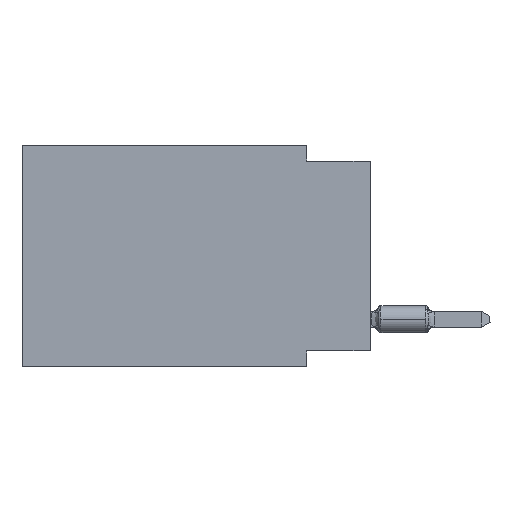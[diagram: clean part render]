
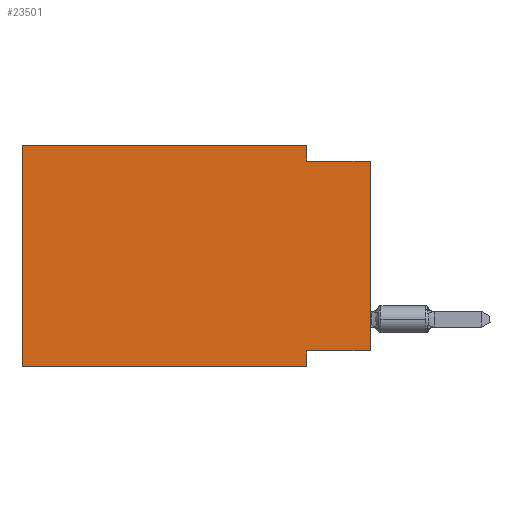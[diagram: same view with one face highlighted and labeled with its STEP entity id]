
A CAD part, left-side view. The second image highlights one B-rep face of the part: STEP entity #23501.
In plain terms, the highlighted planar face has unit normal (-1, 0, 0).
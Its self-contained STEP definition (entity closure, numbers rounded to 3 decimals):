
#1011 = DIRECTION ( 'NONE',  ( 0., -1., 0. ) ) ;
#1168 = DIRECTION ( 'NONE',  ( 0., -1., 0. ) ) ;
#1797 = FACE_OUTER_BOUND ( 'NONE', #10952, .T. ) ;
#2019 = ORIENTED_EDGE ( 'NONE', *, *, #16806, .T. ) ;
#2637 = CARTESIAN_POINT ( 'NONE',  ( 0., 2.54, -0.635 ) ) ;
#2719 = DIRECTION ( 'NONE',  ( 0., 0., 1. ) ) ;
#2873 = CARTESIAN_POINT ( 'NONE',  ( 0., 13.97, 0. ) ) ;
#3123 = ORIENTED_EDGE ( 'NONE', *, *, #26583, .F. ) ;
#3257 = VECTOR ( 'NONE', #14113, 1000. ) ;
#3931 = LINE ( 'NONE', #24537, #25781 ) ;
#4317 = VECTOR ( 'NONE', #22562, 1000. ) ;
#5229 = VECTOR ( 'NONE', #2719, 1000. ) ;
#5337 = LINE ( 'NONE', #26248, #3257 ) ;
#5746 = VERTEX_POINT ( 'NONE', #18652 ) ;
#6087 = ORIENTED_EDGE ( 'NONE', *, *, #20131, .F. ) ;
#6376 = CARTESIAN_POINT ( 'NONE',  ( 0., 0., -8.255 ) ) ;
#6647 = LINE ( 'NONE', #29732, #27024 ) ;
#6682 = DIRECTION ( 'NONE',  ( 0., 1., 0. ) ) ;
#6787 = EDGE_CURVE ( 'NONE', #20504, #18149, #25435, .T. ) ;
#6939 = DIRECTION ( 'NONE',  ( 0., 0., 1. ) ) ;
#8239 = VERTEX_POINT ( 'NONE', #13643 ) ;
#9642 = CARTESIAN_POINT ( 'NONE',  ( 0., 0., 0. ) ) ;
#10952 = EDGE_LOOP ( 'NONE', ( #2019, #6087, #3123, #14873, #24690, #19203, #22703, #20435 ) ) ;
#11014 = EDGE_CURVE ( 'NONE', #18149, #5746, #6647, .T. ) ;
#13643 = CARTESIAN_POINT ( 'NONE',  ( 0., 0., -0.635 ) ) ;
#14113 = DIRECTION ( 'NONE',  ( 0., 0., -1. ) ) ;
#14243 = AXIS2_PLACEMENT_3D ( 'NONE', #14782, #18091, #25171 ) ;
#14412 = LINE ( 'NONE', #9642, #5229 ) ;
#14782 = CARTESIAN_POINT ( 'NONE',  ( 0., 13.97, 0. ) ) ;
#14873 = ORIENTED_EDGE ( 'NONE', *, *, #24060, .F. ) ;
#15031 = LINE ( 'NONE', #22084, #24600 ) ;
#15197 = CARTESIAN_POINT ( 'NONE',  ( 0., 13.97, -8.89 ) ) ;
#15259 = VERTEX_POINT ( 'NONE', #20238 ) ;
#16036 = DIRECTION ( 'NONE',  ( 0., 0., -1. ) ) ;
#16806 = EDGE_CURVE ( 'NONE', #20504, #8239, #14412, .T. ) ;
#17033 = LINE ( 'NONE', #15197, #4317 ) ;
#17533 = PLANE ( 'NONE',  #14243 ) ;
#18091 = DIRECTION ( 'NONE',  ( 1., 0., 0. ) ) ;
#18149 = VERTEX_POINT ( 'NONE', #18528 ) ;
#18171 = CARTESIAN_POINT ( 'NONE',  ( 0., 13.97, 0. ) ) ;
#18528 = CARTESIAN_POINT ( 'NONE',  ( 0., 2.54, -8.255 ) ) ;
#18652 = CARTESIAN_POINT ( 'NONE',  ( 0., 2.54, -8.89 ) ) ;
#19007 = VERTEX_POINT ( 'NONE', #25108 ) ;
#19043 = VERTEX_POINT ( 'NONE', #2637 ) ;
#19203 = ORIENTED_EDGE ( 'NONE', *, *, #27958, .T. ) ;
#20131 = EDGE_CURVE ( 'NONE', #19043, #8239, #3931, .T. ) ;
#20238 = CARTESIAN_POINT ( 'NONE',  ( 0., 13.97, -8.89 ) ) ;
#20435 = ORIENTED_EDGE ( 'NONE', *, *, #6787, .F. ) ;
#20504 = VERTEX_POINT ( 'NONE', #26577 ) ;
#22084 = CARTESIAN_POINT ( 'NONE',  ( 0., 13.97, 0. ) ) ;
#22562 = DIRECTION ( 'NONE',  ( 0., -1., 0. ) ) ;
#22703 = ORIENTED_EDGE ( 'NONE', *, *, #11014, .F. ) ;
#23274 = EDGE_CURVE ( 'NONE', #15259, #25084, #27720, .T. ) ;
#23501 = ADVANCED_FACE ( 'NONE', ( #1797 ), #17533, .F. ) ;
#24060 = EDGE_CURVE ( 'NONE', #25084, #19007, #15031, .T. ) ;
#24537 = CARTESIAN_POINT ( 'NONE',  ( 0., 0., -0.635 ) ) ;
#24600 = VECTOR ( 'NONE', #1011, 1000. ) ;
#24690 = ORIENTED_EDGE ( 'NONE', *, *, #23274, .F. ) ;
#25084 = VERTEX_POINT ( 'NONE', #2873 ) ;
#25108 = CARTESIAN_POINT ( 'NONE',  ( 0., 2.54, 0. ) ) ;
#25171 = DIRECTION ( 'NONE',  ( 0., 0., -1. ) ) ;
#25435 = LINE ( 'NONE', #6376, #26061 ) ;
#25781 = VECTOR ( 'NONE', #1168, 1000. ) ;
#26061 = VECTOR ( 'NONE', #6682, 1000. ) ;
#26248 = CARTESIAN_POINT ( 'NONE',  ( 0., 2.54, 0. ) ) ;
#26577 = CARTESIAN_POINT ( 'NONE',  ( 0., 0., -8.255 ) ) ;
#26583 = EDGE_CURVE ( 'NONE', #19007, #19043, #5337, .T. ) ;
#27024 = VECTOR ( 'NONE', #16036, 1000. ) ;
#27720 = LINE ( 'NONE', #18171, #29458 ) ;
#27958 = EDGE_CURVE ( 'NONE', #15259, #5746, #17033, .T. ) ;
#29458 = VECTOR ( 'NONE', #6939, 1000. ) ;
#29732 = CARTESIAN_POINT ( 'NONE',  ( 0., 2.54, -8.89 ) ) ;
